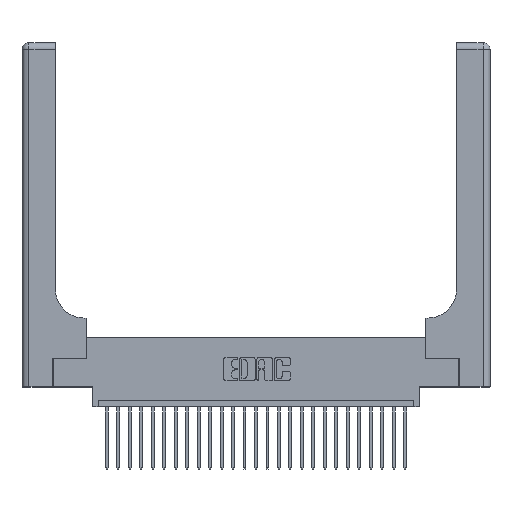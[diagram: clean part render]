
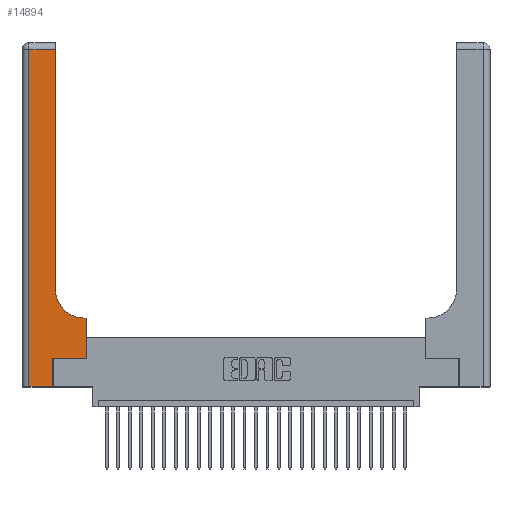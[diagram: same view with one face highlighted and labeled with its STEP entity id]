
A CAD part, top view. The second image highlights one B-rep face of the part: STEP entity #14894.
In plain terms, the highlighted planar face has unit normal (0, 0, 1).
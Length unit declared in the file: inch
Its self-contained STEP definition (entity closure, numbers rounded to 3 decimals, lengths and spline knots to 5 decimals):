
#22 = VERTEX_POINT ( 'NONE', #16377 ) ;
#517 = CARTESIAN_POINT ( 'NONE',  ( 0.06, 3., 0.37 ) ) ;
#1447 = LINE ( 'NONE', #14888, #20159 ) ;
#1457 = LINE ( 'NONE', #4186, #16872 ) ;
#1651 = ORIENTED_EDGE ( 'NONE', *, *, #25932, .T. ) ;
#1745 = PLANE ( 'NONE',  #24762 ) ;
#2285 = EDGE_CURVE ( 'NONE', #20294, #12363, #1447, .T. ) ;
#2334 = LINE ( 'NONE', #24595, #17058 ) ;
#2934 = CARTESIAN_POINT ( 'NONE',  ( 0.5585, 0.25, 0.37 ) ) ;
#3280 = CARTESIAN_POINT ( 'NONE',  ( 0.06, 0., 0.37 ) ) ;
#3356 = EDGE_CURVE ( 'NONE', #9557, #15271, #5721, .T. ) ;
#3637 = VECTOR ( 'NONE', #24146, 39.37008 ) ;
#3719 = DIRECTION ( 'NONE',  ( -1., 0., 0. ) ) ;
#4186 = CARTESIAN_POINT ( 'NONE',  ( 0.5585, 0.25, 0.37 ) ) ;
#4831 = LINE ( 'NONE', #6110, #20546 ) ;
#4864 = VECTOR ( 'NONE', #5002, 39.37008 ) ;
#5002 = DIRECTION ( 'NONE',  ( -1., 0., 0. ) ) ;
#5226 = CARTESIAN_POINT ( 'NONE',  ( 0.5415, 0.85, 0.37 ) ) ;
#5575 = LINE ( 'NONE', #517, #23620 ) ;
#5663 = EDGE_CURVE ( 'NONE', #22, #9549, #17346, .T. ) ;
#5721 = LINE ( 'NONE', #6195, #21417 ) ;
#5763 = ORIENTED_EDGE ( 'NONE', *, *, #6978, .T. ) ;
#6110 = CARTESIAN_POINT ( 'NONE',  ( 0., 0., 0.37 ) ) ;
#6195 = CARTESIAN_POINT ( 'NONE',  ( 0.269, 0., 0.37 ) ) ;
#6978 = EDGE_CURVE ( 'NONE', #27125, #14150, #5575, .T. ) ;
#7475 = ORIENTED_EDGE ( 'NONE', *, *, #15016, .T. ) ;
#9263 = DIRECTION ( 'NONE',  ( 0., -1., 0. ) ) ;
#9404 = DIRECTION ( 'NONE',  ( 0., 0., -1. ) ) ;
#9549 = VERTEX_POINT ( 'NONE', #12098 ) ;
#9557 = VERTEX_POINT ( 'NONE', #23023 ) ;
#9958 = ORIENTED_EDGE ( 'NONE', *, *, #3356, .T. ) ;
#10171 = FACE_OUTER_BOUND ( 'NONE', #25069, .T. ) ;
#10528 = LINE ( 'NONE', #26122, #4864 ) ;
#10709 = CARTESIAN_POINT ( 'NONE',  ( 0.269, 0.25, 0.37 ) ) ;
#10815 = DIRECTION ( 'NONE',  ( 0., 1., 0. ) ) ;
#11792 = DIRECTION ( 'NONE',  ( 1., 0., 0. ) ) ;
#12098 = CARTESIAN_POINT ( 'NONE',  ( 0.5415, 0.6, 0.37 ) ) ;
#12363 = VERTEX_POINT ( 'NONE', #14815 ) ;
#14150 = VERTEX_POINT ( 'NONE', #3280 ) ;
#14591 = ORIENTED_EDGE ( 'NONE', *, *, #20542, .T. ) ;
#14815 = CARTESIAN_POINT ( 'NONE',  ( 0.2915, 2.94, 0.37 ) ) ;
#14888 = CARTESIAN_POINT ( 'NONE',  ( 0.2915, 3., 0.37 ) ) ;
#14894 = ADVANCED_FACE ( 'NONE', ( #10171 ), #1745, .F. ) ;
#15016 = EDGE_CURVE ( 'NONE', #14150, #9557, #4831, .T. ) ;
#15247 = AXIS2_PLACEMENT_3D ( 'NONE', #5226, #9404, #20183 ) ;
#15271 = VERTEX_POINT ( 'NONE', #10709 ) ;
#15333 = EDGE_CURVE ( 'NONE', #22429, #22, #1457, .T. ) ;
#16249 = CARTESIAN_POINT ( 'NONE',  ( 0.2915, 0.85, 0.37 ) ) ;
#16377 = CARTESIAN_POINT ( 'NONE',  ( 0.5585, 0.6, 0.37 ) ) ;
#16693 = DIRECTION ( 'NONE',  ( 0., 0., -1. ) ) ;
#16872 = VECTOR ( 'NONE', #21187, 39.37008 ) ;
#17058 = VECTOR ( 'NONE', #11792, 39.37008 ) ;
#17346 = LINE ( 'NONE', #22168, #3637 ) ;
#18152 = EDGE_CURVE ( 'NONE', #15271, #22429, #2334, .T. ) ;
#18742 = ORIENTED_EDGE ( 'NONE', *, *, #18152, .T. ) ;
#19499 = CARTESIAN_POINT ( 'NONE',  ( 0.06, 2.94, 0.37 ) ) ;
#20159 = VECTOR ( 'NONE', #10815, 39.37008 ) ;
#20183 = DIRECTION ( 'NONE',  ( 1., 0., 0. ) ) ;
#20294 = VERTEX_POINT ( 'NONE', #16249 ) ;
#20542 = EDGE_CURVE ( 'NONE', #12363, #27125, #10528, .T. ) ;
#20546 = VECTOR ( 'NONE', #25376, 39.37008 ) ;
#20974 = DIRECTION ( 'NONE',  ( 0., 1., 0. ) ) ;
#20980 = CARTESIAN_POINT ( 'NONE',  ( 0., 3., 0.37 ) ) ;
#21003 = CIRCLE ( 'NONE', #15247, 0.25 ) ;
#21025 = ORIENTED_EDGE ( 'NONE', *, *, #5663, .T. ) ;
#21187 = DIRECTION ( 'NONE',  ( 0., 1., 0. ) ) ;
#21417 = VECTOR ( 'NONE', #20974, 39.37008 ) ;
#22168 = CARTESIAN_POINT ( 'NONE',  ( 0.2915, 0.6, 0.37 ) ) ;
#22429 = VERTEX_POINT ( 'NONE', #2934 ) ;
#23023 = CARTESIAN_POINT ( 'NONE',  ( 0.269, 0., 0.37 ) ) ;
#23620 = VECTOR ( 'NONE', #9263, 39.37008 ) ;
#24146 = DIRECTION ( 'NONE',  ( -1., 0., 0. ) ) ;
#24595 = CARTESIAN_POINT ( 'NONE',  ( 0.269, 0.25, 0.37 ) ) ;
#24694 = ORIENTED_EDGE ( 'NONE', *, *, #2285, .T. ) ;
#24762 = AXIS2_PLACEMENT_3D ( 'NONE', #20980, #16693, #3719 ) ;
#25069 = EDGE_LOOP ( 'NONE', ( #24694, #14591, #5763, #7475, #9958, #18742, #26278, #21025, #1651 ) ) ;
#25376 = DIRECTION ( 'NONE',  ( 1., 0., 0. ) ) ;
#25932 = EDGE_CURVE ( 'NONE', #9549, #20294, #21003, .T. ) ;
#26122 = CARTESIAN_POINT ( 'NONE',  ( 0., 2.94, 0.37 ) ) ;
#26278 = ORIENTED_EDGE ( 'NONE', *, *, #15333, .T. ) ;
#27125 = VERTEX_POINT ( 'NONE', #19499 ) ;
